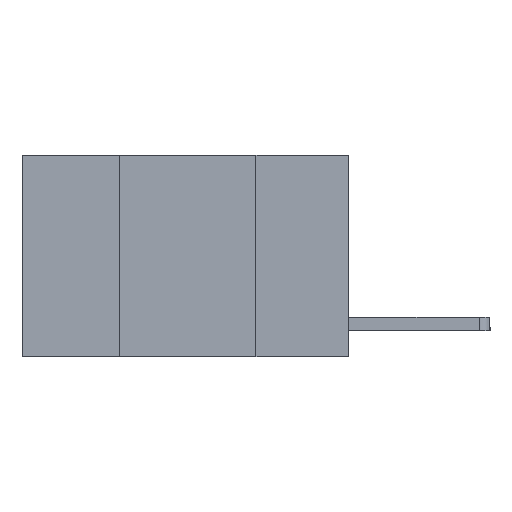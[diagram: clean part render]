
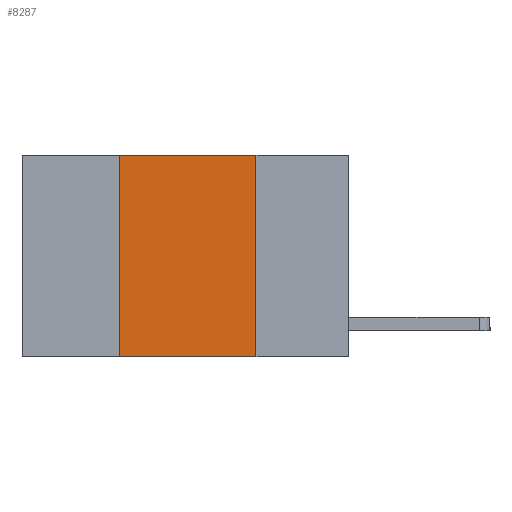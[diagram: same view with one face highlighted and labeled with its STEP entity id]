
A CAD part, left-side view. The second image highlights one B-rep face of the part: STEP entity #8287.
In plain terms, the highlighted planar face has unit normal (-1, 0, 0).
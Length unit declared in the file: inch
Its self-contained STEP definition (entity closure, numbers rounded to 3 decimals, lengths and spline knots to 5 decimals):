
#59 = DIRECTION ( 'NONE',  ( 0., 0., 1. ) ) ;
#155 = CARTESIAN_POINT ( 'NONE',  ( 0., 0.6, 0. ) ) ;
#481 = VERTEX_POINT ( 'NONE', #9530 ) ;
#647 = LINE ( 'NONE', #2995, #4954 ) ;
#758 = PLANE ( 'NONE',  #1237 ) ;
#783 = ORIENTED_EDGE ( 'NONE', *, *, #3174, .F. ) ;
#818 = EDGE_LOOP ( 'NONE', ( #3832, #5306, #783, #7826 ) ) ;
#865 = CARTESIAN_POINT ( 'NONE',  ( 0., 0.42, -0.37 ) ) ;
#1237 = AXIS2_PLACEMENT_3D ( 'NONE', #7038, #9389, #3869 ) ;
#2472 = VERTEX_POINT ( 'NONE', #10080 ) ;
#2760 = LINE ( 'NONE', #5776, #2796 ) ;
#2796 = VECTOR ( 'NONE', #8111, 39.37008 ) ;
#2995 = CARTESIAN_POINT ( 'NONE',  ( 0., 0.6, -0.37 ) ) ;
#3174 = EDGE_CURVE ( 'NONE', #8855, #7089, #6219, .T. ) ;
#3343 = EDGE_CURVE ( 'NONE', #2472, #481, #2760, .T. ) ;
#3570 = EDGE_CURVE ( 'NONE', #7089, #2472, #7901, .T. ) ;
#3832 = ORIENTED_EDGE ( 'NONE', *, *, #3343, .F. ) ;
#3869 = DIRECTION ( 'NONE',  ( 0., 0., -1. ) ) ;
#4307 = VECTOR ( 'NONE', #4840, 39.37008 ) ;
#4635 = FACE_OUTER_BOUND ( 'NONE', #818, .T. ) ;
#4840 = DIRECTION ( 'NONE',  ( 0., -1., 0. ) ) ;
#4954 = VECTOR ( 'NONE', #5191, 39.37008 ) ;
#5191 = DIRECTION ( 'NONE',  ( 0., -1., 0. ) ) ;
#5306 = ORIENTED_EDGE ( 'NONE', *, *, #3570, .F. ) ;
#5776 = CARTESIAN_POINT ( 'NONE',  ( 0., 0.17, 0. ) ) ;
#6219 = LINE ( 'NONE', #6381, #9974 ) ;
#6381 = CARTESIAN_POINT ( 'NONE',  ( 0., 0.42, 0. ) ) ;
#7038 = CARTESIAN_POINT ( 'NONE',  ( 0., 0.6, 0. ) ) ;
#7089 = VERTEX_POINT ( 'NONE', #9199 ) ;
#7350 = EDGE_CURVE ( 'NONE', #8855, #481, #647, .T. ) ;
#7826 = ORIENTED_EDGE ( 'NONE', *, *, #7350, .T. ) ;
#7901 = LINE ( 'NONE', #155, #4307 ) ;
#8111 = DIRECTION ( 'NONE',  ( 0., 0., -1. ) ) ;
#8287 = ADVANCED_FACE ( 'NONE', ( #4635 ), #758, .F. ) ;
#8855 = VERTEX_POINT ( 'NONE', #865 ) ;
#9199 = CARTESIAN_POINT ( 'NONE',  ( 0., 0.42, 0. ) ) ;
#9389 = DIRECTION ( 'NONE',  ( 1., 0., 0. ) ) ;
#9530 = CARTESIAN_POINT ( 'NONE',  ( 0., 0.17, -0.37 ) ) ;
#9974 = VECTOR ( 'NONE', #59, 39.37008 ) ;
#10080 = CARTESIAN_POINT ( 'NONE',  ( 0., 0.17, 0. ) ) ;
